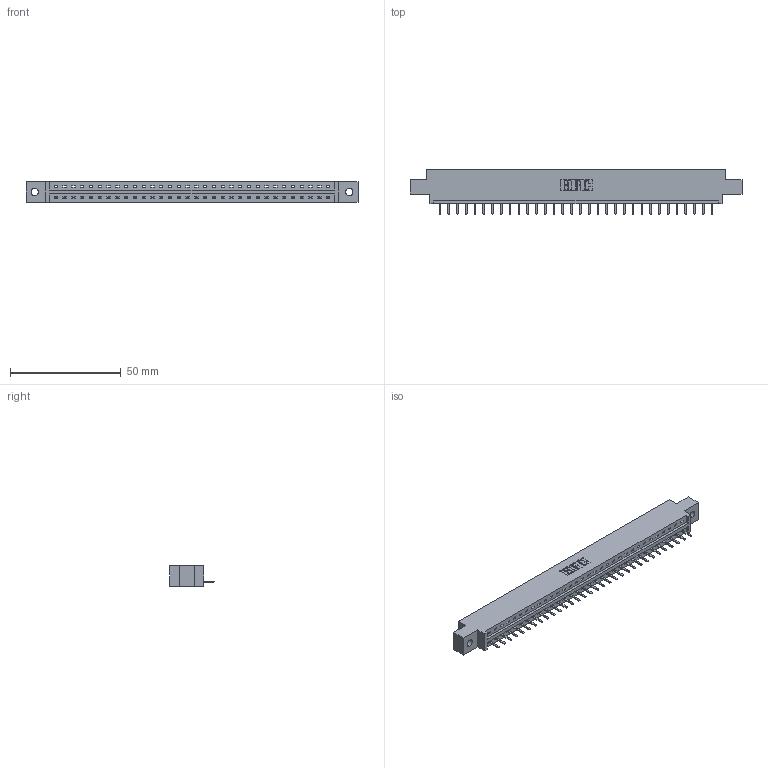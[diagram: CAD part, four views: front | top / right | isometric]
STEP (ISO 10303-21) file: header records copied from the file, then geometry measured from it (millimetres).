
FILE_DESCRIPTION (( 'STEP AP203' ), '1' );
FILE_NAME ('387-032-520-602.STEP', '2019-10-03T20:05:54', ( '' ), ( '' ), 'SwSTEP 2.0', 'SolidWorks 2016', '' );
FILE_SCHEMA (( 'CONFIG_CONTROL_DESIGN' ));
Length unit declared in the file: inch
Products named in the file (3): 345-292-001_345-293-120; 387-032-520-602; 337 Part_0.170 Offset - 0.128 Dia
Assembly tree (33 placements, depth 2):
  387-032-520-602
    337 Part_0.170 Offset - 0.128 Dia
    345-292-001_345-293-120  x32
Bounding box: 149.81 x 20.02 x 9.4 mm (x, y, z)
Volume: 15198.8 mm3; surface area: 15145.4 mm2
Topology: 33 solids, 33 shells, 2230 faces, 6595 edges, 4310 vertices
Faces by surface type: plane 1610, cylinder 620
Entity records: 25329 total; most frequent: CARTESIAN_POINT 4430, ORIENTED_EDGE 4386, DIRECTION 3737, EDGE_CURVE 2193, LINE 2061, VECTOR 2061, VERTEX_POINT 1458, AXIS2_PLACEMENT_3D 838
